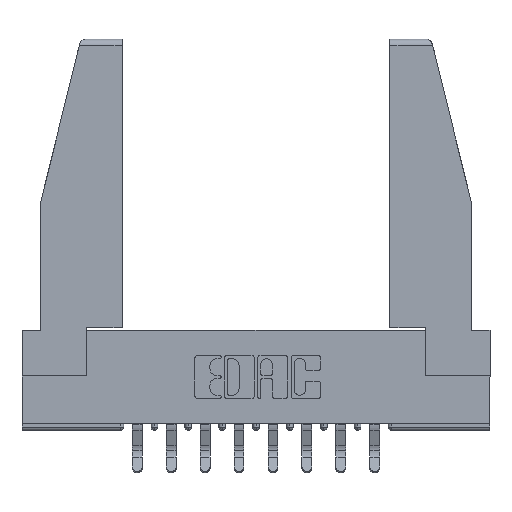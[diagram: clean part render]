
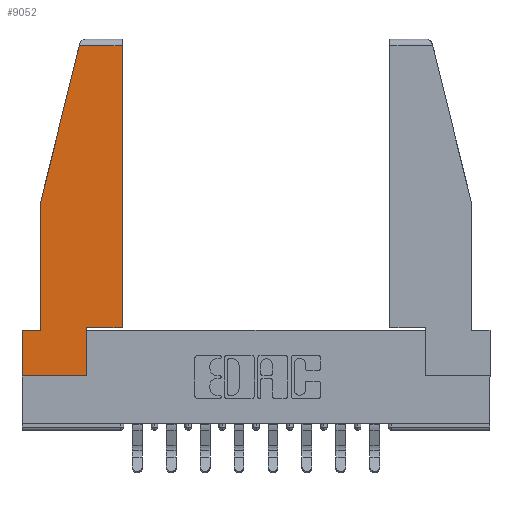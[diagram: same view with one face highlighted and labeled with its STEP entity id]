
A CAD part, top view. The second image highlights one B-rep face of the part: STEP entity #9052.
In plain terms, the highlighted planar face has unit normal (0, 0, 1).
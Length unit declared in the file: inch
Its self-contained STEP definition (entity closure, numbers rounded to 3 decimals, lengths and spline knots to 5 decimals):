
#52 = CARTESIAN_POINT ( 'NONE',  ( 0.086, 0.8, 0. ) ) ;
#86 = DIRECTION ( 'NONE',  ( -1., 0., 0. ) ) ;
#191 = CARTESIAN_POINT ( 'NONE',  ( 0., 0., 0. ) ) ;
#192 = DIRECTION ( 'NONE',  ( 1., 0., 0. ) ) ;
#225 = CARTESIAN_POINT ( 'NONE',  ( 0.297, 0., 0. ) ) ;
#245 = CARTESIAN_POINT ( 'NONE',  ( 0., 0., 0. ) ) ;
#278 = EDGE_CURVE ( 'NONE', #6477, #9728, #5150, .T. ) ;
#511 = PLANE ( 'NONE',  #10994 ) ;
#558 = DIRECTION ( 'NONE',  ( 1., 0., 0. ) ) ;
#863 = LINE ( 'NONE', #9391, #4041 ) ;
#1123 = VECTOR ( 'NONE', #15491, 39.37008 ) ;
#1277 = VECTOR ( 'NONE', #9958, 39.37008 ) ;
#1608 = CARTESIAN_POINT ( 'NONE',  ( 0.297, 0.223, 0. ) ) ;
#1773 = LINE ( 'NONE', #12006, #3283 ) ;
#2456 = LINE ( 'NONE', #2509, #12739 ) ;
#2509 = CARTESIAN_POINT ( 'NONE',  ( 0., 0.21, 0. ) ) ;
#2699 = ORIENTED_EDGE ( 'NONE', *, *, #6756, .T. ) ;
#2869 = VERTEX_POINT ( 'NONE', #13794 ) ;
#3279 = VERTEX_POINT ( 'NONE', #8052 ) ;
#3283 = VECTOR ( 'NONE', #86, 39.37008 ) ;
#3448 = CARTESIAN_POINT ( 'NONE',  ( 0., 0.21, 0. ) ) ;
#3542 = VERTEX_POINT ( 'NONE', #7174 ) ;
#3569 = ORIENTED_EDGE ( 'NONE', *, *, #10982, .T. ) ;
#3717 = VERTEX_POINT ( 'NONE', #8385 ) ;
#4000 = ORIENTED_EDGE ( 'NONE', *, *, #7913, .T. ) ;
#4041 = VECTOR ( 'NONE', #12843, 39.37008 ) ;
#4084 = ORIENTED_EDGE ( 'NONE', *, *, #278, .T. ) ;
#4463 = LINE ( 'NONE', #1608, #1277 ) ;
#5150 = LINE ( 'NONE', #245, #7383 ) ;
#5367 = VERTEX_POINT ( 'NONE', #12498 ) ;
#5517 = EDGE_CURVE ( 'NONE', #2869, #6477, #10377, .T. ) ;
#5536 = EDGE_CURVE ( 'NONE', #5367, #14967, #863, .T. ) ;
#5767 = EDGE_CURVE ( 'NONE', #3717, #5367, #1773, .T. ) ;
#5770 = CARTESIAN_POINT ( 'NONE',  ( 0.086, 0.8, 0. ) ) ;
#5830 = DIRECTION ( 'NONE',  ( 0., -1., 0. ) ) ;
#5940 = DIRECTION ( 'NONE',  ( 0., -1., 0. ) ) ;
#6332 = DIRECTION ( 'NONE',  ( 0., 0., 1. ) ) ;
#6369 = ORIENTED_EDGE ( 'NONE', *, *, #7439, .T. ) ;
#6477 = VERTEX_POINT ( 'NONE', #191 ) ;
#6708 = ORIENTED_EDGE ( 'NONE', *, *, #5517, .T. ) ;
#6756 = EDGE_CURVE ( 'NONE', #3279, #2869, #2456, .T. ) ;
#7144 = DIRECTION ( 'NONE',  ( -1., 0., 0. ) ) ;
#7174 = CARTESIAN_POINT ( 'NONE',  ( 0.461, 0.223, 0. ) ) ;
#7383 = VECTOR ( 'NONE', #192, 39.37008 ) ;
#7439 = EDGE_CURVE ( 'NONE', #14967, #3279, #15155, .T. ) ;
#7677 = CARTESIAN_POINT ( 'NONE',  ( 0., 0., 0. ) ) ;
#7780 = FACE_OUTER_BOUND ( 'NONE', #15199, .T. ) ;
#7913 = EDGE_CURVE ( 'NONE', #3542, #3717, #12882, .T. ) ;
#8052 = CARTESIAN_POINT ( 'NONE',  ( 0.086, 0.21, 0. ) ) ;
#8195 = VECTOR ( 'NONE', #5940, 39.37008 ) ;
#8316 = ORIENTED_EDGE ( 'NONE', *, *, #5767, .T. ) ;
#8355 = CARTESIAN_POINT ( 'NONE',  ( 0.461, 0.223, 0. ) ) ;
#8385 = CARTESIAN_POINT ( 'NONE',  ( 0.461, 1.52, 0. ) ) ;
#8689 = CARTESIAN_POINT ( 'NONE',  ( 0.297, 0., 0. ) ) ;
#8879 = VECTOR ( 'NONE', #11281, 39.37008 ) ;
#8986 = EDGE_CURVE ( 'NONE', #9823, #3542, #4463, .T. ) ;
#9052 = ADVANCED_FACE ( 'NONE', ( #7780 ), #511, .T. ) ;
#9391 = CARTESIAN_POINT ( 'NONE',  ( 0.271, 1.55, 0. ) ) ;
#9728 = VERTEX_POINT ( 'NONE', #225 ) ;
#9820 = VECTOR ( 'NONE', #5830, 39.37008 ) ;
#9823 = VERTEX_POINT ( 'NONE', #11131 ) ;
#9958 = DIRECTION ( 'NONE',  ( 1., 0., 0. ) ) ;
#10377 = LINE ( 'NONE', #3448, #9820 ) ;
#10484 = ORIENTED_EDGE ( 'NONE', *, *, #8986, .T. ) ;
#10982 = EDGE_CURVE ( 'NONE', #9728, #9823, #11699, .T. ) ;
#10994 = AXIS2_PLACEMENT_3D ( 'NONE', #7677, #6332, #558 ) ;
#11041 = ORIENTED_EDGE ( 'NONE', *, *, #5536, .T. ) ;
#11131 = CARTESIAN_POINT ( 'NONE',  ( 0.297, 0.223, 0. ) ) ;
#11281 = DIRECTION ( 'NONE',  ( 0., 1., 0. ) ) ;
#11699 = LINE ( 'NONE', #8689, #8879 ) ;
#12006 = CARTESIAN_POINT ( 'NONE',  ( 0., 1.52, 0. ) ) ;
#12498 = CARTESIAN_POINT ( 'NONE',  ( 0.2636, 1.52, 0. ) ) ;
#12739 = VECTOR ( 'NONE', #7144, 39.37008 ) ;
#12843 = DIRECTION ( 'NONE',  ( -0.239, -0.971, 0. ) ) ;
#12882 = LINE ( 'NONE', #8355, #1123 ) ;
#13794 = CARTESIAN_POINT ( 'NONE',  ( 0., 0.21, 0. ) ) ;
#14967 = VERTEX_POINT ( 'NONE', #52 ) ;
#15155 = LINE ( 'NONE', #5770, #8195 ) ;
#15199 = EDGE_LOOP ( 'NONE', ( #4000, #8316, #11041, #6369, #2699, #6708, #4084, #3569, #10484 ) ) ;
#15491 = DIRECTION ( 'NONE',  ( 0., 1., 0. ) ) ;
